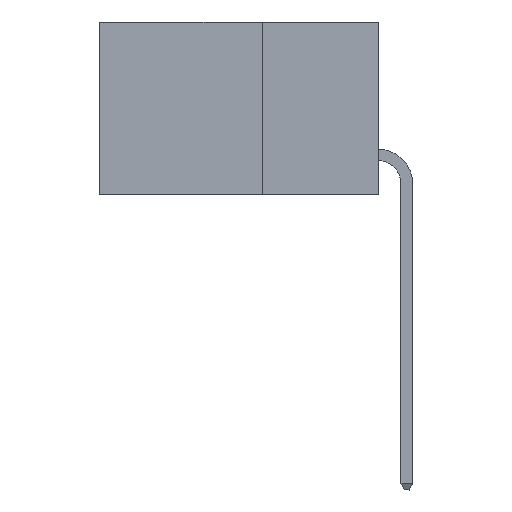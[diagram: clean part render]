
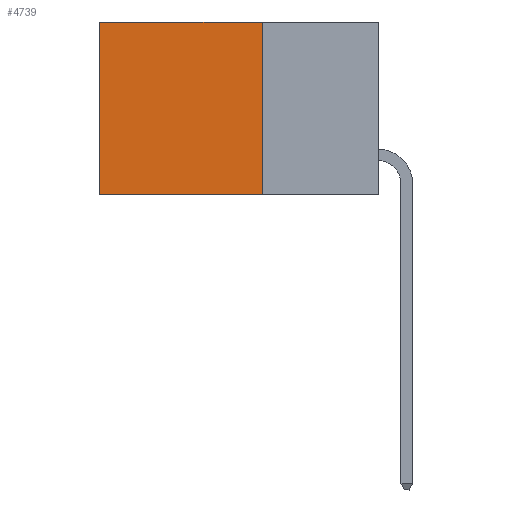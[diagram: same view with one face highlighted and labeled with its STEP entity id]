
A CAD part, left-side view. The second image highlights one B-rep face of the part: STEP entity #4739.
In plain terms, the highlighted planar face has unit normal (-1, 0, 0).
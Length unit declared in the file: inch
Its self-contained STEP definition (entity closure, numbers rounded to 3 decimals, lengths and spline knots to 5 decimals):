
#300 = VECTOR ( 'NONE', #7627, 39.37008 ) ;
#663 = VERTEX_POINT ( 'NONE', #14609 ) ;
#1018 = VERTEX_POINT ( 'NONE', #14953 ) ;
#1744 = EDGE_CURVE ( 'NONE', #663, #1018, #6930, .T. ) ;
#2437 = EDGE_LOOP ( 'NONE', ( #15677, #10375, #6706, #9401 ) ) ;
#2570 = EDGE_CURVE ( 'NONE', #13720, #663, #8134, .T. ) ;
#3057 = EDGE_CURVE ( 'NONE', #3504, #1018, #6878, .T. ) ;
#3169 = EDGE_CURVE ( 'NONE', #13720, #3504, #8739, .T. ) ;
#3391 = CARTESIAN_POINT ( 'NONE',  ( 0.298, 0.6, 0. ) ) ;
#3504 = VERTEX_POINT ( 'NONE', #9026 ) ;
#4100 = DIRECTION ( 'NONE',  ( 0., 0., -1. ) ) ;
#4739 = ADVANCED_FACE ( 'NONE', ( #10304 ), #8959, .F. ) ;
#6706 = ORIENTED_EDGE ( 'NONE', *, *, #2570, .F. ) ;
#6878 = LINE ( 'NONE', #3391, #9944 ) ;
#6930 = LINE ( 'NONE', #9854, #300 ) ;
#7627 = DIRECTION ( 'NONE',  ( 0., 1., 0. ) ) ;
#7865 = CARTESIAN_POINT ( 'NONE',  ( 0.298, 0.25, 0. ) ) ;
#8134 = LINE ( 'NONE', #15947, #10371 ) ;
#8319 = VECTOR ( 'NONE', #13872, 39.37008 ) ;
#8385 = DIRECTION ( 'NONE',  ( 0., 0., -1. ) ) ;
#8410 = DIRECTION ( 'NONE',  ( 1., 0., 0. ) ) ;
#8469 = CARTESIAN_POINT ( 'NONE',  ( 0.298, 0.25, 0. ) ) ;
#8739 = LINE ( 'NONE', #10216, #8319 ) ;
#8959 = PLANE ( 'NONE',  #16348 ) ;
#9026 = CARTESIAN_POINT ( 'NONE',  ( 0.298, 0.6, 0. ) ) ;
#9401 = ORIENTED_EDGE ( 'NONE', *, *, #3169, .T. ) ;
#9854 = CARTESIAN_POINT ( 'NONE',  ( 0.298, 0.25, -0.37 ) ) ;
#9944 = VECTOR ( 'NONE', #4100, 39.37008 ) ;
#10216 = CARTESIAN_POINT ( 'NONE',  ( 0.298, 0.25, 0. ) ) ;
#10304 = FACE_OUTER_BOUND ( 'NONE', #2437, .T. ) ;
#10371 = VECTOR ( 'NONE', #16053, 39.37008 ) ;
#10375 = ORIENTED_EDGE ( 'NONE', *, *, #1744, .F. ) ;
#13720 = VERTEX_POINT ( 'NONE', #7865 ) ;
#13872 = DIRECTION ( 'NONE',  ( 0., 1., 0. ) ) ;
#14609 = CARTESIAN_POINT ( 'NONE',  ( 0.298, 0.25, -0.37 ) ) ;
#14953 = CARTESIAN_POINT ( 'NONE',  ( 0.298, 0.6, -0.37 ) ) ;
#15677 = ORIENTED_EDGE ( 'NONE', *, *, #3057, .T. ) ;
#15947 = CARTESIAN_POINT ( 'NONE',  ( 0.298, 0.25, 0. ) ) ;
#16053 = DIRECTION ( 'NONE',  ( 0., 0., -1. ) ) ;
#16348 = AXIS2_PLACEMENT_3D ( 'NONE', #8469, #8410, #8385 ) ;
